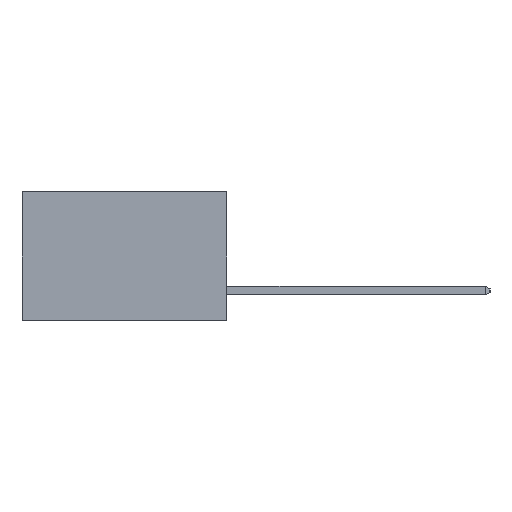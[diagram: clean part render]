
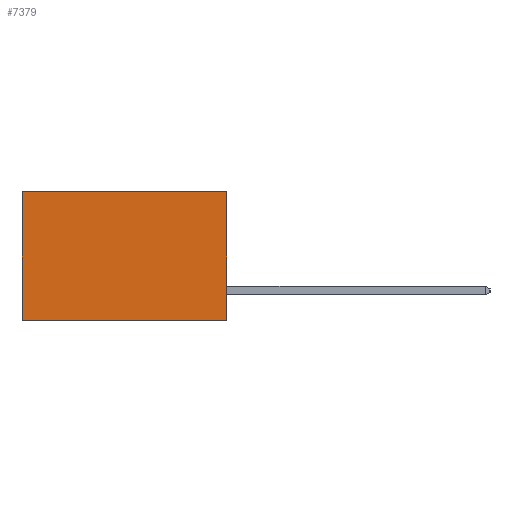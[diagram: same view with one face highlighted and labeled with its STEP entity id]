
A CAD part, left-side view. The second image highlights one B-rep face of the part: STEP entity #7379.
In plain terms, the highlighted planar face has unit normal (-1, 0, 0).
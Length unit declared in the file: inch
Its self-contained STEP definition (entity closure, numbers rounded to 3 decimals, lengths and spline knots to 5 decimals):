
#1012 = LINE ( 'NONE', #4297, #5295 ) ;
#3620 = FACE_OUTER_BOUND ( 'NONE', #5348, .T. ) ;
#3834 = VECTOR ( 'NONE', #16061, 39.37008 ) ;
#4276 = DIRECTION ( 'NONE',  ( 0., 0., -1. ) ) ;
#4297 = CARTESIAN_POINT ( 'NONE',  ( 0.277, 0., -0.37 ) ) ;
#5295 = VECTOR ( 'NONE', #4276, 39.37008 ) ;
#5348 = EDGE_LOOP ( 'NONE', ( #12785, #17863, #15106, #13078 ) ) ;
#5355 = CARTESIAN_POINT ( 'NONE',  ( 0.277, 0.59, 0. ) ) ;
#5481 = VERTEX_POINT ( 'NONE', #11089 ) ;
#5694 = DIRECTION ( 'NONE',  ( 0., 1., 0. ) ) ;
#6469 = CARTESIAN_POINT ( 'NONE',  ( 0.277, 0.59, -0.37 ) ) ;
#7379 = ADVANCED_FACE ( 'NONE', ( #3620 ), #12319, .F. ) ;
#7738 = EDGE_CURVE ( 'NONE', #8969, #5481, #1012, .T. ) ;
#8740 = EDGE_CURVE ( 'NONE', #22677, #9290, #13352, .T. ) ;
#8969 = VERTEX_POINT ( 'NONE', #12005 ) ;
#9290 = VERTEX_POINT ( 'NONE', #6469 ) ;
#9600 = AXIS2_PLACEMENT_3D ( 'NONE', #12418, #12540, #12207 ) ;
#10334 = LINE ( 'NONE', #14505, #13870 ) ;
#11089 = CARTESIAN_POINT ( 'NONE',  ( 0.277, 0., -0.37 ) ) ;
#12005 = CARTESIAN_POINT ( 'NONE',  ( 0.277, 0., 0. ) ) ;
#12207 = DIRECTION ( 'NONE',  ( 0., 0., -1. ) ) ;
#12319 = PLANE ( 'NONE',  #9600 ) ;
#12418 = CARTESIAN_POINT ( 'NONE',  ( 0.277, 0., -0.37 ) ) ;
#12540 = DIRECTION ( 'NONE',  ( 1., 0., 0. ) ) ;
#12785 = ORIENTED_EDGE ( 'NONE', *, *, #8740, .T. ) ;
#13078 = ORIENTED_EDGE ( 'NONE', *, *, #22159, .T. ) ;
#13352 = LINE ( 'NONE', #16166, #3834 ) ;
#13870 = VECTOR ( 'NONE', #5694, 39.37008 ) ;
#14505 = CARTESIAN_POINT ( 'NONE',  ( 0.277, 0., 0. ) ) ;
#15106 = ORIENTED_EDGE ( 'NONE', *, *, #7738, .F. ) ;
#16061 = DIRECTION ( 'NONE',  ( 0., 0., -1. ) ) ;
#16166 = CARTESIAN_POINT ( 'NONE',  ( 0.277, 0.59, -0.37 ) ) ;
#16859 = VECTOR ( 'NONE', #18701, 39.37008 ) ;
#17011 = CARTESIAN_POINT ( 'NONE',  ( 0.277, 0., -0.37 ) ) ;
#17863 = ORIENTED_EDGE ( 'NONE', *, *, #21005, .F. ) ;
#18701 = DIRECTION ( 'NONE',  ( 0., 1., 0. ) ) ;
#21005 = EDGE_CURVE ( 'NONE', #5481, #9290, #21312, .T. ) ;
#21312 = LINE ( 'NONE', #17011, #16859 ) ;
#22159 = EDGE_CURVE ( 'NONE', #8969, #22677, #10334, .T. ) ;
#22677 = VERTEX_POINT ( 'NONE', #5355 ) ;
